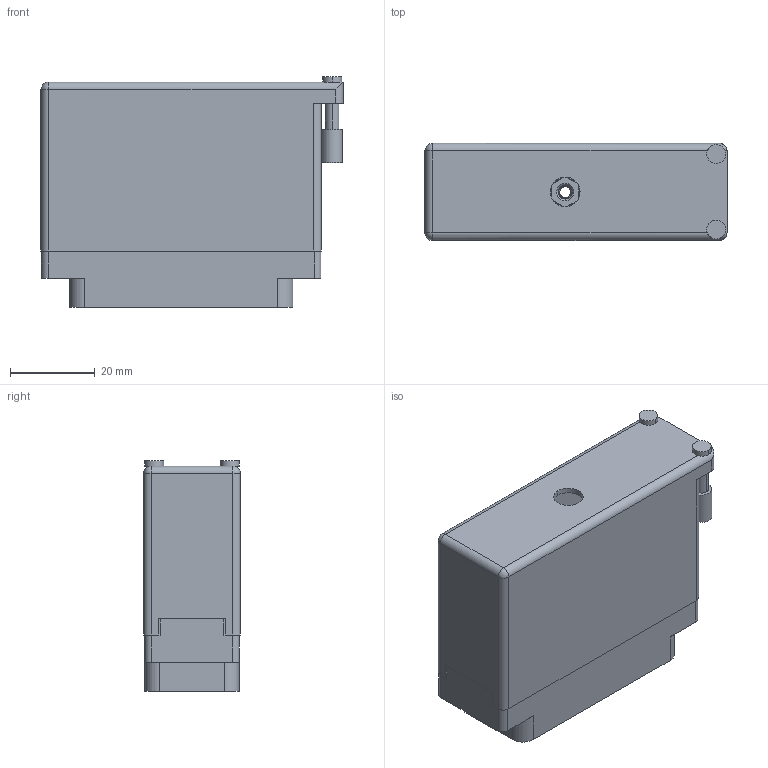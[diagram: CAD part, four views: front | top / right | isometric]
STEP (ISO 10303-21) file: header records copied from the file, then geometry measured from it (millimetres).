
FILE_DESCRIPTION (( 'STEP AP203' ), '1' );
FILE_NAME ('516-056-000-356.STEP', '2020-03-10T04:49:56', ( '' ), ( '' ), 'SwSTEP 2.0', 'SolidWorks 2016', '' );
FILE_SCHEMA (( 'CONFIG_CONTROL_DESIGN' ));
Length unit declared in the file: inch
Products named in the file (4): 516-230-001_Metal - 056 Side Entry; 516 Plug Insulator_056; 516-252-035-100_516-252-035-100; 516-056-000-356
Assembly tree (3 placements, depth 2):
  516-056-000-356
    516 Plug Insulator_056
    516-230-001_Metal - 056 Side Entry
    516-252-035-100_516-252-035-100
Bounding box: 71.12 x 22.83 x 54.31 mm (x, y, z)
Volume: 22002.9 mm3; surface area: 32168.7 mm2
Topology: 3 solids, 3 shells, 1333 faces, 3901 edges, 2592 vertices
Faces by surface type: plane 941, cylinder 372, cone 12, bspline 6, sphere 2
Entity records: 47161 total; most frequent: CARTESIAN_POINT 10317, ORIENTED_EDGE 7798, DIRECTION 7463, EDGE_CURVE 3899, LINE 2891, VECTOR 2891, VERTEX_POINT 2592, AXIS2_PLACEMENT_3D 2286
